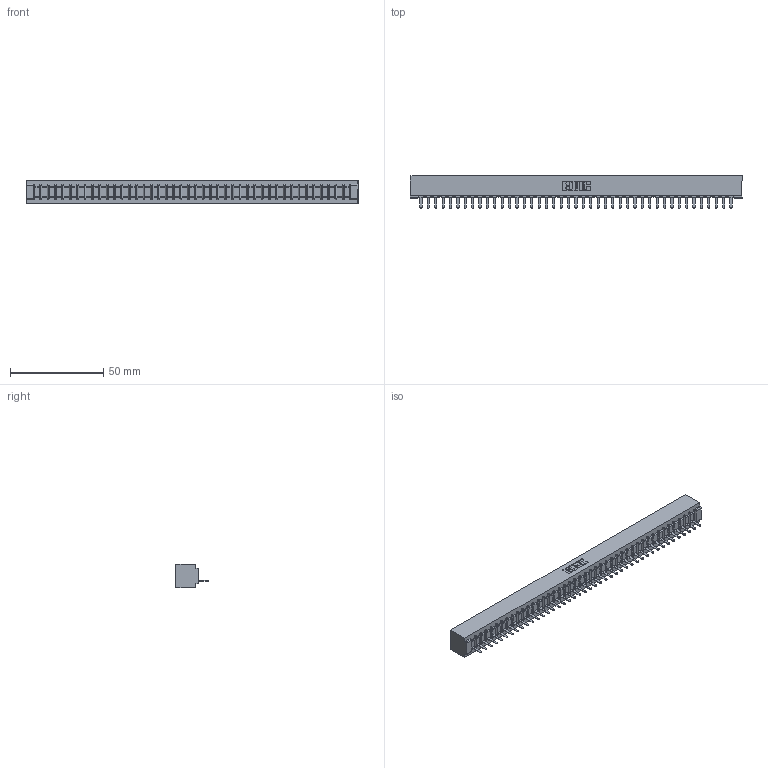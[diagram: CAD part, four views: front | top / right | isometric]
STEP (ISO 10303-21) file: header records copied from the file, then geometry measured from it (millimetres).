
FILE_DESCRIPTION (( 'STEP AP203' ), '1' );
FILE_NAME ('357-043-421-101.STEP', '2020-10-03T13:09:26', ( '' ), ( '' ), 'SwSTEP 2.0', 'SolidWorks 2020', '' );
FILE_SCHEMA (( 'CONFIG_CONTROL_DESIGN' ));
Length unit declared in the file: inch
Products named in the file (3): 307-290-002_521; 307 Part_No Mounting Lugs; 357-043-421-101
Assembly tree (44 placements, depth 2):
  357-043-421-101
    307 Part_No Mounting Lugs
    307-290-002_521  x43
Bounding box: 178.26 x 17.42 x 12.7 mm (x, y, z)
Volume: 19643.5 mm3; surface area: 25077.5 mm2
Topology: 44 solids, 44 shells, 3336 faces, 10275 edges, 6730 vertices
Faces by surface type: plane 2001, cylinder 1247, sphere 88
Entity records: 37180 total; most frequent: CARTESIAN_POINT 6272, ORIENTED_EDGE 6262, DIRECTION 6091, EDGE_CURVE 3131, VECTOR 2401, LINE 2401, VERTEX_POINT 2026, AXIS2_PLACEMENT_3D 1845
